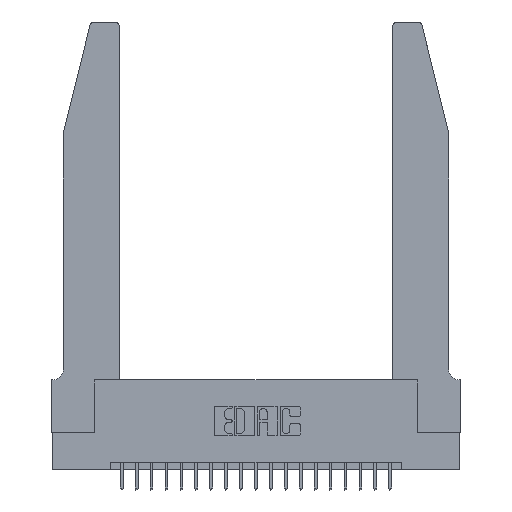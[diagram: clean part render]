
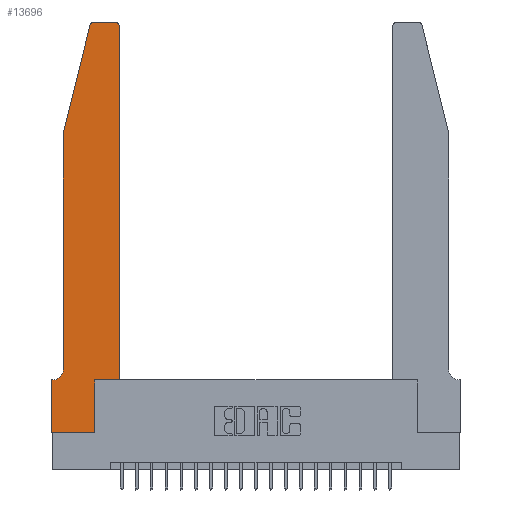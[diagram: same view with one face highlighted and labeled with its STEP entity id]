
A CAD part, top view. The second image highlights one B-rep face of the part: STEP entity #13696.
In plain terms, the highlighted planar face has unit normal (0, 0, 1).
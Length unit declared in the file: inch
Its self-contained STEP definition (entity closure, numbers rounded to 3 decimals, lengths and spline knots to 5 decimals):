
#167 = VECTOR ( 'NONE', #2642, 39.37008 ) ;
#246 = CARTESIAN_POINT ( 'NONE',  ( 0.0755, 0.35, 0.37 ) ) ;
#342 = FACE_OUTER_BOUND ( 'NONE', #10454, .T. ) ;
#375 = CARTESIAN_POINT ( 'NONE',  ( 0.4205, 2.75, 0.37 ) ) ;
#385 = ORIENTED_EDGE ( 'NONE', *, *, #17732, .T. ) ;
#491 = VERTEX_POINT ( 'NONE', #14801 ) ;
#580 = VERTEX_POINT ( 'NONE', #3125 ) ;
#621 = ORIENTED_EDGE ( 'NONE', *, *, #4443, .T. ) ;
#721 = VERTEX_POINT ( 'NONE', #2074 ) ;
#732 = CARTESIAN_POINT ( 'NONE',  ( 0.4205, 2.72, 0.37 ) ) ;
#1042 = CARTESIAN_POINT ( 'NONE',  ( 0., 0., 0.37 ) ) ;
#1079 = DIRECTION ( 'NONE',  ( 0., 1., 0. ) ) ;
#1173 = VERTEX_POINT ( 'NONE', #20052 ) ;
#1313 = LINE ( 'NONE', #8420, #7927 ) ;
#1510 = VERTEX_POINT ( 'NONE', #3394 ) ;
#1625 = EDGE_CURVE ( 'NONE', #1173, #580, #5700, .T. ) ;
#2073 = EDGE_CURVE ( 'NONE', #580, #13599, #16628, .T. ) ;
#2074 = CARTESIAN_POINT ( 'NONE',  ( 0.0755, 2., 0.37 ) ) ;
#2453 = EDGE_CURVE ( 'NONE', #19109, #1173, #13526, .T. ) ;
#2642 = DIRECTION ( 'NONE',  ( 0., -1., 0. ) ) ;
#2896 = LINE ( 'NONE', #1042, #6063 ) ;
#3086 = EDGE_CURVE ( 'NONE', #7177, #1510, #6060, .T. ) ;
#3125 = CARTESIAN_POINT ( 'NONE',  ( 0., 0.35, 0.37 ) ) ;
#3394 = CARTESIAN_POINT ( 'NONE',  ( 0.25487, 2.72718, 0.37 ) ) ;
#3824 = CARTESIAN_POINT ( 'NONE',  ( 0., 0.35, 0.37 ) ) ;
#4204 = ORIENTED_EDGE ( 'NONE', *, *, #16472, .T. ) ;
#4284 = CARTESIAN_POINT ( 'NONE',  ( 0., 0., 0.37 ) ) ;
#4428 = AXIS2_PLACEMENT_3D ( 'NONE', #732, #7837, #21344 ) ;
#4443 = EDGE_CURVE ( 'NONE', #19049, #7177, #8224, .T. ) ;
#4719 = DIRECTION ( 'NONE',  ( -1., 0., 0. ) ) ;
#5119 = DIRECTION ( 'NONE',  ( 0., 0., 1. ) ) ;
#5175 = CIRCLE ( 'NONE', #4428, 0.03 ) ;
#5502 = LINE ( 'NONE', #12436, #11959 ) ;
#5700 = LINE ( 'NONE', #246, #16353 ) ;
#6060 = CIRCLE ( 'NONE', #18964, 0.03 ) ;
#6063 = VECTOR ( 'NONE', #15142, 39.37008 ) ;
#7177 = VERTEX_POINT ( 'NONE', #15438 ) ;
#7400 = CARTESIAN_POINT ( 'NONE',  ( 0.0055, 0.42, 0.37 ) ) ;
#7671 = DIRECTION ( 'NONE',  ( 0., 0., 1. ) ) ;
#7837 = DIRECTION ( 'NONE',  ( 0., 0., 1. ) ) ;
#7927 = VECTOR ( 'NONE', #21930, 39.37008 ) ;
#8224 = LINE ( 'NONE', #20566, #21998 ) ;
#8337 = VERTEX_POINT ( 'NONE', #8859 ) ;
#8420 = CARTESIAN_POINT ( 'NONE',  ( 0.0755, 2., 0.37 ) ) ;
#8859 = CARTESIAN_POINT ( 'NONE',  ( 0.4505, 2.72, 0.37 ) ) ;
#9263 = DIRECTION ( 'NONE',  ( 0., 0., -1. ) ) ;
#9683 = ORIENTED_EDGE ( 'NONE', *, *, #18388, .T. ) ;
#9741 = VECTOR ( 'NONE', #17772, 39.37008 ) ;
#10224 = DIRECTION ( 'NONE',  ( 1., 0., 0. ) ) ;
#10454 = EDGE_LOOP ( 'NONE', ( #621, #12447, #16207, #4204, #15086, #20305, #17985, #9683, #21553, #385, #10570, #20646 ) ) ;
#10570 = ORIENTED_EDGE ( 'NONE', *, *, #16972, .T. ) ;
#10736 = VECTOR ( 'NONE', #1079, 39.37008 ) ;
#10761 = LINE ( 'NONE', #14433, #9741 ) ;
#11059 = EDGE_CURVE ( 'NONE', #8337, #19049, #5175, .T. ) ;
#11247 = DIRECTION ( 'NONE',  ( -1., 0., 0. ) ) ;
#11804 = CARTESIAN_POINT ( 'NONE',  ( 0.0755, 2., 0.37 ) ) ;
#11857 = EDGE_CURVE ( 'NONE', #491, #16349, #20525, .T. ) ;
#11959 = VECTOR ( 'NONE', #19481, 39.37008 ) ;
#12054 = CARTESIAN_POINT ( 'NONE',  ( 0.284, 2.72, 0.37 ) ) ;
#12436 = CARTESIAN_POINT ( 'NONE',  ( 0.4505, 0.35, 0.37 ) ) ;
#12447 = ORIENTED_EDGE ( 'NONE', *, *, #3086, .T. ) ;
#13361 = AXIS2_PLACEMENT_3D ( 'NONE', #3824, #7671, #16180 ) ;
#13526 = CIRCLE ( 'NONE', #21652, 0.07 ) ;
#13599 = VERTEX_POINT ( 'NONE', #21635 ) ;
#13696 = ADVANCED_FACE ( 'NONE', ( #342 ), #16398, .T. ) ;
#14415 = DIRECTION ( 'NONE',  ( -1., 0., 0. ) ) ;
#14433 = CARTESIAN_POINT ( 'NONE',  ( 0.4505, 0.35, 0.37 ) ) ;
#14801 = CARTESIAN_POINT ( 'NONE',  ( 0.2865, 0., 0.37 ) ) ;
#15086 = ORIENTED_EDGE ( 'NONE', *, *, #2453, .T. ) ;
#15142 = DIRECTION ( 'NONE',  ( 1., 0., 0. ) ) ;
#15438 = CARTESIAN_POINT ( 'NONE',  ( 0.284, 2.75, 0.37 ) ) ;
#15586 = EDGE_CURVE ( 'NONE', #1510, #721, #22334, .T. ) ;
#16180 = DIRECTION ( 'NONE',  ( 1., 0., 0. ) ) ;
#16207 = ORIENTED_EDGE ( 'NONE', *, *, #15586, .T. ) ;
#16349 = VERTEX_POINT ( 'NONE', #20194 ) ;
#16353 = VECTOR ( 'NONE', #11247, 39.37008 ) ;
#16398 = PLANE ( 'NONE',  #13361 ) ;
#16472 = EDGE_CURVE ( 'NONE', #721, #19109, #1313, .T. ) ;
#16628 = LINE ( 'NONE', #4284, #167 ) ;
#16972 = EDGE_CURVE ( 'NONE', #18888, #8337, #10761, .T. ) ;
#17040 = CARTESIAN_POINT ( 'NONE',  ( 0.4505, 0.35, 0.37 ) ) ;
#17732 = EDGE_CURVE ( 'NONE', #16349, #18888, #5502, .T. ) ;
#17772 = DIRECTION ( 'NONE',  ( 0., 1., 0. ) ) ;
#17985 = ORIENTED_EDGE ( 'NONE', *, *, #2073, .T. ) ;
#18388 = EDGE_CURVE ( 'NONE', #13599, #491, #2896, .T. ) ;
#18589 = VECTOR ( 'NONE', #20484, 39.37008 ) ;
#18888 = VERTEX_POINT ( 'NONE', #17040 ) ;
#18964 = AXIS2_PLACEMENT_3D ( 'NONE', #12054, #5119, #10224 ) ;
#19049 = VERTEX_POINT ( 'NONE', #375 ) ;
#19109 = VERTEX_POINT ( 'NONE', #19942 ) ;
#19481 = DIRECTION ( 'NONE',  ( 1., 0., 0. ) ) ;
#19942 = CARTESIAN_POINT ( 'NONE',  ( 0.0755, 0.42, 0.37 ) ) ;
#20052 = CARTESIAN_POINT ( 'NONE',  ( 0.0055, 0.35, 0.37 ) ) ;
#20194 = CARTESIAN_POINT ( 'NONE',  ( 0.2865, 0.35, 0.37 ) ) ;
#20305 = ORIENTED_EDGE ( 'NONE', *, *, #1625, .T. ) ;
#20484 = DIRECTION ( 'NONE',  ( -0.239, -0.971, 0. ) ) ;
#20525 = LINE ( 'NONE', #22261, #10736 ) ;
#20566 = CARTESIAN_POINT ( 'NONE',  ( 0.2605, 2.75, 0.37 ) ) ;
#20646 = ORIENTED_EDGE ( 'NONE', *, *, #11059, .T. ) ;
#21344 = DIRECTION ( 'NONE',  ( 1., 0., 0. ) ) ;
#21553 = ORIENTED_EDGE ( 'NONE', *, *, #11857, .T. ) ;
#21635 = CARTESIAN_POINT ( 'NONE',  ( 0., 0., 0.37 ) ) ;
#21652 = AXIS2_PLACEMENT_3D ( 'NONE', #7400, #9263, #14415 ) ;
#21930 = DIRECTION ( 'NONE',  ( 0., -1., 0. ) ) ;
#21998 = VECTOR ( 'NONE', #4719, 39.37008 ) ;
#22261 = CARTESIAN_POINT ( 'NONE',  ( 0.2865, 0.35, 0.37 ) ) ;
#22334 = LINE ( 'NONE', #11804, #18589 ) ;
